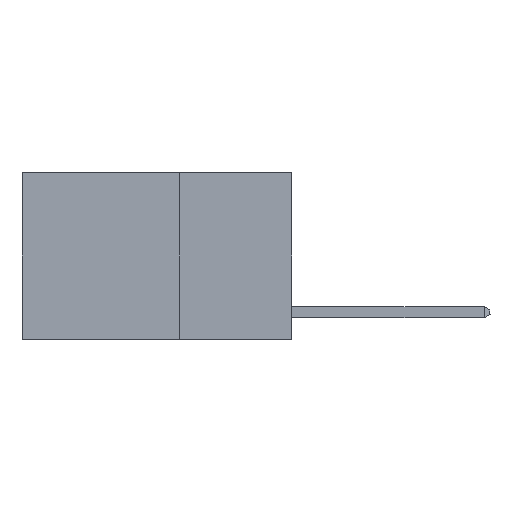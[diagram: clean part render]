
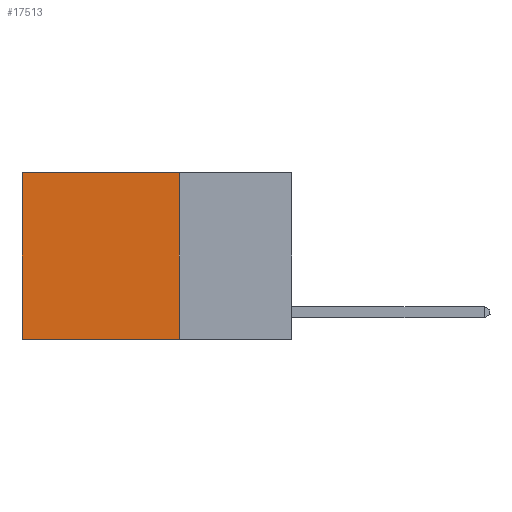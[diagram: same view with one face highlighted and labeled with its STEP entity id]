
A CAD part, left-side view. The second image highlights one B-rep face of the part: STEP entity #17513.
In plain terms, the highlighted planar face has unit normal (-1, 0, 0).
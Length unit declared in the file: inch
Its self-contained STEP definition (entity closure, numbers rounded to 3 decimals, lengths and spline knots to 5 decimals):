
#1069 = CARTESIAN_POINT ( 'NONE',  ( 0.2625, 0.25, 0. ) ) ;
#1221 = VECTOR ( 'NONE', #2293, 39.37008 ) ;
#1272 = DIRECTION ( 'NONE',  ( 0., 1., 0. ) ) ;
#1328 = CARTESIAN_POINT ( 'NONE',  ( 0.2625, 0.6, 0. ) ) ;
#1634 = LINE ( 'NONE', #6988, #16208 ) ;
#1657 = LINE ( 'NONE', #9509, #1221 ) ;
#2046 = LINE ( 'NONE', #14342, #12752 ) ;
#2293 = DIRECTION ( 'NONE',  ( 0., 0., -1. ) ) ;
#2335 = VERTEX_POINT ( 'NONE', #1069 ) ;
#3189 = CARTESIAN_POINT ( 'NONE',  ( 0.2625, 0.25, 0. ) ) ;
#3549 = FACE_OUTER_BOUND ( 'NONE', #16530, .T. ) ;
#4669 = DIRECTION ( 'NONE',  ( 0., 1., 0. ) ) ;
#6112 = DIRECTION ( 'NONE',  ( 0., 0., -1. ) ) ;
#6988 = CARTESIAN_POINT ( 'NONE',  ( 0.2625, 0.25, 0. ) ) ;
#7265 = ORIENTED_EDGE ( 'NONE', *, *, #16128, .T. ) ;
#7514 = PLANE ( 'NONE',  #17016 ) ;
#7884 = ORIENTED_EDGE ( 'NONE', *, *, #12225, .T. ) ;
#8109 = CARTESIAN_POINT ( 'NONE',  ( 0.2625, 0.25, -0.37 ) ) ;
#8368 = ORIENTED_EDGE ( 'NONE', *, *, #10875, .F. ) ;
#8927 = VECTOR ( 'NONE', #4669, 39.37008 ) ;
#9050 = CARTESIAN_POINT ( 'NONE',  ( 0.2625, 0.25, -0.37 ) ) ;
#9509 = CARTESIAN_POINT ( 'NONE',  ( 0.2625, 0.6, 0. ) ) ;
#9974 = VERTEX_POINT ( 'NONE', #1328 ) ;
#10875 = EDGE_CURVE ( 'NONE', #14017, #14285, #17625, .T. ) ;
#12225 = EDGE_CURVE ( 'NONE', #9974, #14285, #1657, .T. ) ;
#12752 = VECTOR ( 'NONE', #15826, 39.37008 ) ;
#13560 = EDGE_CURVE ( 'NONE', #2335, #14017, #2046, .T. ) ;
#14017 = VERTEX_POINT ( 'NONE', #8109 ) ;
#14285 = VERTEX_POINT ( 'NONE', #14622 ) ;
#14342 = CARTESIAN_POINT ( 'NONE',  ( 0.2625, 0.25, 0. ) ) ;
#14622 = CARTESIAN_POINT ( 'NONE',  ( 0.2625, 0.6, -0.37 ) ) ;
#14874 = DIRECTION ( 'NONE',  ( 1., 0., 0. ) ) ;
#15826 = DIRECTION ( 'NONE',  ( 0., 0., -1. ) ) ;
#16128 = EDGE_CURVE ( 'NONE', #2335, #9974, #1634, .T. ) ;
#16208 = VECTOR ( 'NONE', #1272, 39.37008 ) ;
#16530 = EDGE_LOOP ( 'NONE', ( #7884, #8368, #16829, #7265 ) ) ;
#16829 = ORIENTED_EDGE ( 'NONE', *, *, #13560, .F. ) ;
#17016 = AXIS2_PLACEMENT_3D ( 'NONE', #3189, #14874, #6112 ) ;
#17513 = ADVANCED_FACE ( 'NONE', ( #3549 ), #7514, .F. ) ;
#17625 = LINE ( 'NONE', #9050, #8927 ) ;
